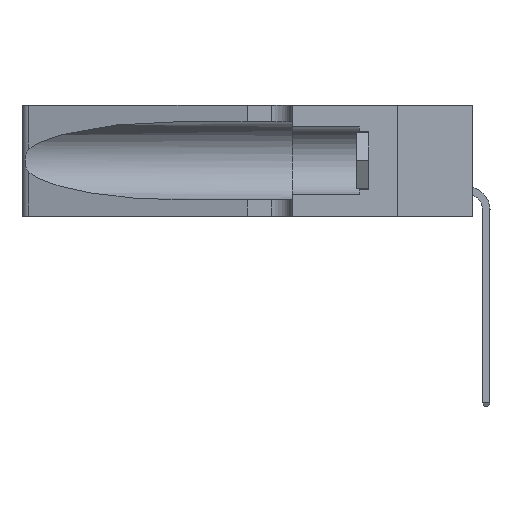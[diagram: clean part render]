
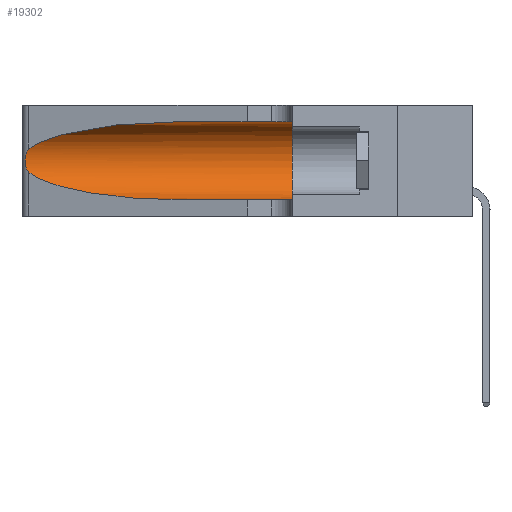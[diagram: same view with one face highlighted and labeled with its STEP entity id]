
A CAD part, left-side view. The second image highlights one B-rep face of the part: STEP entity #19302.
In plain terms, the highlighted cylindrical face has radius 3.308 mm (diameter 6.617 mm), a partial arc.
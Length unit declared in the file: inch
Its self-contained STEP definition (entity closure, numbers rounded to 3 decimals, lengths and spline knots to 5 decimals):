
#740 = CARTESIAN_POINT ( 'NONE',  ( 0.25487, 1.22718, 0.14631 ) ) ;
#1227 = CARTESIAN_POINT ( 'NONE',  ( 0.25487, 1.22718, 0.22369 ) ) ;
#1648 = EDGE_LOOP ( 'NONE', ( #15940, #6474, #18055, #28452, #19562, #3142 ) ) ;
#1790 =( BOUNDED_CURVE ( )  B_SPLINE_CURVE ( 3, ( #22913, #25240, #11869, #20973 ),
 .UNSPECIFIED., .F., .F. ) 
 B_SPLINE_CURVE_WITH_KNOTS ( ( 4, 4 ),
 ( 3.44316, 4.71239 ),
 .UNSPECIFIED. ) 
 CURVE ( )  GEOMETRIC_REPRESENTATION_ITEM ( )  RATIONAL_B_SPLINE_CURVE ( ( 1., 0.87, 0.87, 1. ) ) 
 REPRESENTATION_ITEM ( '' )  );
#2373 = CARTESIAN_POINT ( 'NONE',  ( 0.26075, 1.23896, 0.19203 ) ) ;
#2567 = VERTEX_POINT ( 'NONE', #19543 ) ;
#2691 = LINE ( 'NONE', #25905, #13615 ) ;
#3142 = ORIENTED_EDGE ( 'NONE', *, *, #13822, .F. ) ;
#3533 = VERTEX_POINT ( 'NONE', #1227 ) ;
#4073 = VERTEX_POINT ( 'NONE', #11679 ) ;
#4668 = EDGE_CURVE ( 'NONE', #23716, #2567, #2691, .T. ) ;
#4758 = VECTOR ( 'NONE', #6898, 39.37008 ) ;
#4812 = CARTESIAN_POINT ( 'NONE',  ( 0.25789, 1.23486, 0.15765 ) ) ;
#6170 = CARTESIAN_POINT ( 'NONE',  ( 0.1305, 0.72297, 0.05475 ) ) ;
#6474 = ORIENTED_EDGE ( 'NONE', *, *, #22393, .T. ) ;
#6795 = CARTESIAN_POINT ( 'NONE',  ( 0.25854, 1.2359, 0.20912 ) ) ;
#6898 = DIRECTION ( 'NONE',  ( 0., -1., 0. ) ) ;
#8132 = DIRECTION ( 'NONE',  ( 0., 0., 1. ) ) ;
#8216 = EDGE_CURVE ( 'NONE', #17111, #3533, #22097, .T. ) ;
#8239 = VERTEX_POINT ( 'NONE', #15478 ) ;
#8263 = B_SPLINE_CURVE_WITH_KNOTS ( 'NONE', 3,
 ( #26202, #28484, #20104, #26753, #6795, #11010, #2373, #8961, #11207, #9237, #4812, #22841, #11791, #740 ),
 .UNSPECIFIED., .F., .F.,
 ( 4, 2, 2, 2, 2, 2, 4 ),
 ( 0., 0.00027, 0.00053, 0.00107, 0.0016, 0.00187, 0.00214 ),
 .UNSPECIFIED. ) ;
#8961 = CARTESIAN_POINT ( 'NONE',  ( 0.26075, 1.23896, 0.178 ) ) ;
#9237 = CARTESIAN_POINT ( 'NONE',  ( 0.25856, 1.23593, 0.16098 ) ) ;
#9342 = DIRECTION ( 'NONE',  ( 0., -1., 0. ) ) ;
#10402 = DIRECTION ( 'NONE',  ( 0., 1., 0. ) ) ;
#10967 = CARTESIAN_POINT ( 'NONE',  ( 0.18966, 0.96281, 0.31525 ) ) ;
#11010 = CARTESIAN_POINT ( 'NONE',  ( 0.26018, 1.23835, 0.19895 ) ) ;
#11207 = CARTESIAN_POINT ( 'NONE',  ( 0.26017, 1.23833, 0.17102 ) ) ;
#11679 = CARTESIAN_POINT ( 'NONE',  ( 0.1305, 0.35, 0.31525 ) ) ;
#11791 = CARTESIAN_POINT ( 'NONE',  ( 0.25555, 1.22993, 0.14849 ) ) ;
#11869 = CARTESIAN_POINT ( 'NONE',  ( 0.18966, 0.96281, 0.05475 ) ) ;
#12547 = CARTESIAN_POINT ( 'NONE',  ( 0.1305, 0.72297, 0.31525 ) ) ;
#13615 = VECTOR ( 'NONE', #21897, 39.37008 ) ;
#13822 = EDGE_CURVE ( 'NONE', #17111, #4073, #20897, .T. ) ;
#13846 = CARTESIAN_POINT ( 'NONE',  ( 0.1305, 1.61858, 0.185 ) ) ;
#14527 = AXIS2_PLACEMENT_3D ( 'NONE', #17325, #10402, #8132 ) ;
#15356 = CYLINDRICAL_SURFACE ( 'NONE', #18014, 0.13025 ) ;
#15478 = CARTESIAN_POINT ( 'NONE',  ( 0.25487, 1.22718, 0.14631 ) ) ;
#15731 = CARTESIAN_POINT ( 'NONE',  ( 0.1305, 1.61858, 0.31525 ) ) ;
#15940 = ORIENTED_EDGE ( 'NONE', *, *, #8216, .T. ) ;
#17111 = VERTEX_POINT ( 'NONE', #12547 ) ;
#17325 = CARTESIAN_POINT ( 'NONE',  ( 0.1305, 0.35, 0.185 ) ) ;
#18014 = AXIS2_PLACEMENT_3D ( 'NONE', #13846, #9342, #24970 ) ;
#18055 = ORIENTED_EDGE ( 'NONE', *, *, #20448, .T. ) ;
#19302 = ADVANCED_FACE ( 'NONE', ( #23715 ), #15356, .F. ) ;
#19543 = CARTESIAN_POINT ( 'NONE',  ( 0.1305, 0.35, 0.05475 ) ) ;
#19562 = ORIENTED_EDGE ( 'NONE', *, *, #22022, .F. ) ;
#19880 = CARTESIAN_POINT ( 'NONE',  ( 0.25487, 1.22718, 0.22369 ) ) ;
#20104 = CARTESIAN_POINT ( 'NONE',  ( 0.25639, 1.23184, 0.21858 ) ) ;
#20448 = EDGE_CURVE ( 'NONE', #8239, #23716, #1790, .T. ) ;
#20566 = CIRCLE ( 'NONE', #14527, 0.13025 ) ;
#20897 = LINE ( 'NONE', #15731, #4758 ) ;
#20973 = CARTESIAN_POINT ( 'NONE',  ( 0.1305, 0.72297, 0.05475 ) ) ;
#21897 = DIRECTION ( 'NONE',  ( 0., -1., 0. ) ) ;
#22022 = EDGE_CURVE ( 'NONE', #4073, #2567, #20566, .T. ) ;
#22097 =( BOUNDED_CURVE ( )  B_SPLINE_CURVE ( 3, ( #24350, #10967, #22427, #19880 ),
 .UNSPECIFIED., .F., .F. ) 
 B_SPLINE_CURVE_WITH_KNOTS ( ( 4, 4 ),
 ( 1.5708, 2.84003 ),
 .UNSPECIFIED. ) 
 CURVE ( )  GEOMETRIC_REPRESENTATION_ITEM ( )  RATIONAL_B_SPLINE_CURVE ( ( 1., 0.87, 0.87, 1. ) ) 
 REPRESENTATION_ITEM ( '' )  );
#22393 = EDGE_CURVE ( 'NONE', #3533, #8239, #8263, .T. ) ;
#22427 = CARTESIAN_POINT ( 'NONE',  ( 0.2373, 1.15595, 0.28018 ) ) ;
#22841 = CARTESIAN_POINT ( 'NONE',  ( 0.25639, 1.23186, 0.15144 ) ) ;
#22913 = CARTESIAN_POINT ( 'NONE',  ( 0.25487, 1.22718, 0.14631 ) ) ;
#23715 = FACE_OUTER_BOUND ( 'NONE', #1648, .T. ) ;
#23716 = VERTEX_POINT ( 'NONE', #6170 ) ;
#24350 = CARTESIAN_POINT ( 'NONE',  ( 0.1305, 0.72297, 0.31525 ) ) ;
#24970 = DIRECTION ( 'NONE',  ( 0., 0., -1. ) ) ;
#25240 = CARTESIAN_POINT ( 'NONE',  ( 0.2373, 1.15595, 0.08982 ) ) ;
#25905 = CARTESIAN_POINT ( 'NONE',  ( 0.1305, 1.61858, 0.05475 ) ) ;
#26202 = CARTESIAN_POINT ( 'NONE',  ( 0.25487, 1.22718, 0.22369 ) ) ;
#26753 = CARTESIAN_POINT ( 'NONE',  ( 0.25787, 1.23484, 0.2124 ) ) ;
#28452 = ORIENTED_EDGE ( 'NONE', *, *, #4668, .T. ) ;
#28484 = CARTESIAN_POINT ( 'NONE',  ( 0.25555, 1.22994, 0.2215 ) ) ;
